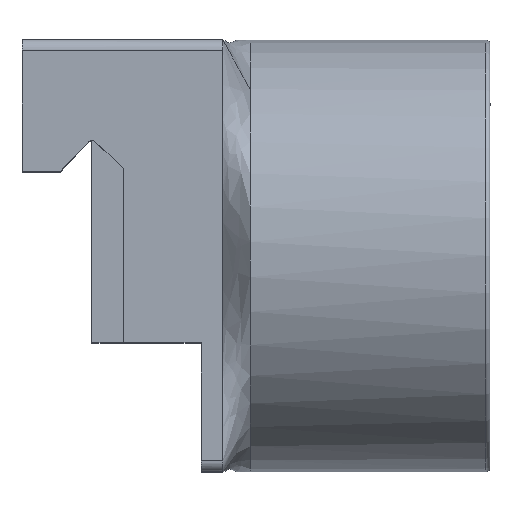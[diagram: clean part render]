
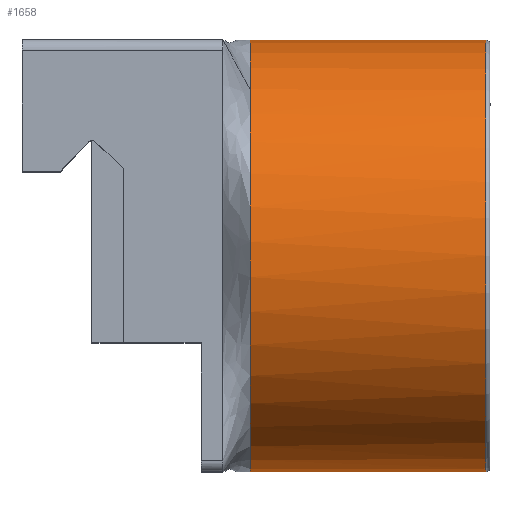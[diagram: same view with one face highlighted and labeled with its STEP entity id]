
A CAD part, top view. The second image highlights one B-rep face of the part: STEP entity #1658.
In plain terms, the highlighted cylindrical face has radius 20 mm (diameter 40 mm), a partial arc.
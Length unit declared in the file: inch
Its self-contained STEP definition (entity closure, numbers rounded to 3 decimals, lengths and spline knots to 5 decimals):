
#70 = AXIS2_PLACEMENT_3D ( 'NONE', #3711, #599, #2466 ) ;
#76 = DIRECTION ( 'NONE',  ( 1., 0., 0. ) ) ;
#459 = VERTEX_POINT ( 'NONE', #1672 ) ;
#599 = DIRECTION ( 'NONE',  ( 1., 0., 0. ) ) ;
#610 = DIRECTION ( 'NONE',  ( 1., 0., 0. ) ) ;
#689 = CARTESIAN_POINT ( 'NONE',  ( 0.83228, -0.18002, -0.18789 ) ) ;
#949 = VERTEX_POINT ( 'NONE', #3246 ) ;
#995 = DIRECTION ( 'NONE',  ( 1., 0., 0. ) ) ;
#1035 = VERTEX_POINT ( 'NONE', #689 ) ;
#1080 = EDGE_CURVE ( 'NONE', #2856, #949, #3252, .T. ) ;
#1383 = CARTESIAN_POINT ( 'NONE',  ( 0.20728, 0., -0.68898 ) ) ;
#1576 = DIRECTION ( 'NONE',  ( -1., 0., 0. ) ) ;
#1658 = ADVANCED_FACE ( 'NONE', ( #3331 ), #2383, .T. ) ;
#1672 = CARTESIAN_POINT ( 'NONE',  ( 0.83228, 0.00001, -0.68898 ) ) ;
#1748 = DIRECTION ( 'NONE',  ( 1., 0., 0. ) ) ;
#1775 = ORIENTED_EDGE ( 'NONE', *, *, #1080, .T. ) ;
#2081 = CIRCLE ( 'NONE', #2631, 0.7874 ) ;
#2253 = LINE ( 'NONE', #1383, #3967 ) ;
#2265 = CIRCLE ( 'NONE', #2542, 0.7874 ) ;
#2383 = CYLINDRICAL_SURFACE ( 'NONE', #70, 0.7874 ) ;
#2466 = DIRECTION ( 'NONE',  ( 0., 1., 0. ) ) ;
#2499 = DIRECTION ( 'NONE',  ( 0., -1., 0. ) ) ;
#2542 = AXIS2_PLACEMENT_3D ( 'NONE', #4362, #1748, #2499 ) ;
#2546 = EDGE_CURVE ( 'NONE', #459, #5662, #2253, .T. ) ;
#2631 = AXIS2_PLACEMENT_3D ( 'NONE', #2815, #1576, #3336 ) ;
#2815 = CARTESIAN_POINT ( 'NONE',  ( 1.69228, -0.7874, -0.68898 ) ) ;
#2856 = VERTEX_POINT ( 'NONE', #5656 ) ;
#3025 = ORIENTED_EDGE ( 'NONE', *, *, #5016, .T. ) ;
#3124 = ORIENTED_EDGE ( 'NONE', *, *, #5614, .T. ) ;
#3190 = AXIS2_PLACEMENT_3D ( 'NONE', #3620, #76, #5318 ) ;
#3246 = CARTESIAN_POINT ( 'NONE',  ( 1.69228, -1.5748, -0.68898 ) ) ;
#3252 = LINE ( 'NONE', #3776, #5715 ) ;
#3331 = FACE_OUTER_BOUND ( 'NONE', #4140, .T. ) ;
#3336 = DIRECTION ( 'NONE',  ( 0., -1., 0. ) ) ;
#3620 = CARTESIAN_POINT ( 'NONE',  ( 0.83228, -0.7874, -0.68898 ) ) ;
#3711 = CARTESIAN_POINT ( 'NONE',  ( 0.20728, -0.7874, -0.68898 ) ) ;
#3776 = CARTESIAN_POINT ( 'NONE',  ( 0.20728, -1.5748, -0.68898 ) ) ;
#3967 = VECTOR ( 'NONE', #995, 39.37008 ) ;
#4140 = EDGE_LOOP ( 'NONE', ( #3124, #1775, #3025, #5303, #4597 ) ) ;
#4207 = CIRCLE ( 'NONE', #3190, 0.7874 ) ;
#4362 = CARTESIAN_POINT ( 'NONE',  ( 0.83228, -0.7874, -0.68898 ) ) ;
#4597 = ORIENTED_EDGE ( 'NONE', *, *, #5120, .T. ) ;
#4879 = CARTESIAN_POINT ( 'NONE',  ( 1.69228, 0., -0.68898 ) ) ;
#5016 = EDGE_CURVE ( 'NONE', #949, #5662, #2081, .T. ) ;
#5120 = EDGE_CURVE ( 'NONE', #459, #1035, #2265, .T. ) ;
#5303 = ORIENTED_EDGE ( 'NONE', *, *, #2546, .F. ) ;
#5318 = DIRECTION ( 'NONE',  ( 0., -1., 0. ) ) ;
#5614 = EDGE_CURVE ( 'NONE', #1035, #2856, #4207, .T. ) ;
#5656 = CARTESIAN_POINT ( 'NONE',  ( 0.83228, -1.57481, -0.68898 ) ) ;
#5662 = VERTEX_POINT ( 'NONE', #4879 ) ;
#5715 = VECTOR ( 'NONE', #610, 39.37008 ) ;
